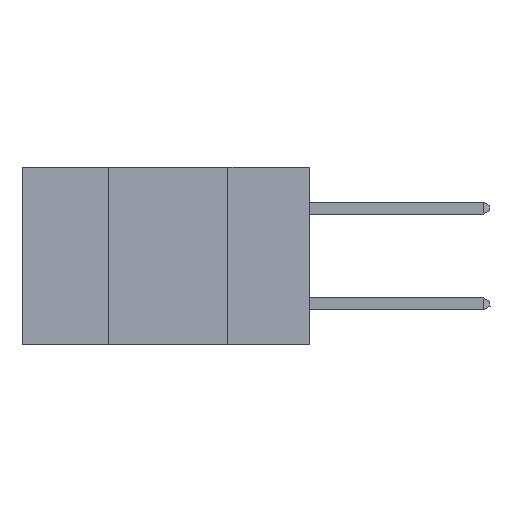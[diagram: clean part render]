
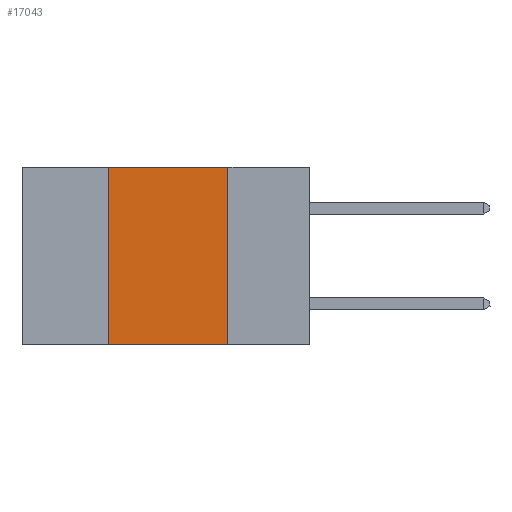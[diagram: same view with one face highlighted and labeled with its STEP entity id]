
A CAD part, left-side view. The second image highlights one B-rep face of the part: STEP entity #17043.
In plain terms, the highlighted planar face has unit normal (-1, 0, 0).
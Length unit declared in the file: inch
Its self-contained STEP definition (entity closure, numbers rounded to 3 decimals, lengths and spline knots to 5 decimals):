
#282 = FACE_OUTER_BOUND ( 'NONE', #10484, .T. ) ;
#453 = ORIENTED_EDGE ( 'NONE', *, *, #3353, .F. ) ;
#843 = EDGE_CURVE ( 'NONE', #7472, #19707, #16392, .T. ) ;
#1840 = VERTEX_POINT ( 'NONE', #17248 ) ;
#2102 = CARTESIAN_POINT ( 'NONE',  ( 0., 0.17, -0.37 ) ) ;
#2778 = CARTESIAN_POINT ( 'NONE',  ( 0., 0.6, -0.37 ) ) ;
#2872 = DIRECTION ( 'NONE',  ( 0., -1., 0. ) ) ;
#3353 = EDGE_CURVE ( 'NONE', #7472, #11350, #10577, .T. ) ;
#3792 = LINE ( 'NONE', #11026, #17487 ) ;
#5064 = CARTESIAN_POINT ( 'NONE',  ( 0., 0.42, 0. ) ) ;
#6886 = DIRECTION ( 'NONE',  ( 0., 0., 1. ) ) ;
#7207 = EDGE_CURVE ( 'NONE', #1840, #19707, #3792, .T. ) ;
#7472 = VERTEX_POINT ( 'NONE', #20380 ) ;
#7990 = DIRECTION ( 'NONE',  ( 1., 0., 0. ) ) ;
#9653 = ORIENTED_EDGE ( 'NONE', *, *, #18401, .F. ) ;
#10167 = CARTESIAN_POINT ( 'NONE',  ( 0., 0.6, 0. ) ) ;
#10215 = ORIENTED_EDGE ( 'NONE', *, *, #843, .T. ) ;
#10484 = EDGE_LOOP ( 'NONE', ( #23046, #9653, #453, #10215 ) ) ;
#10577 = LINE ( 'NONE', #5064, #19283 ) ;
#11026 = CARTESIAN_POINT ( 'NONE',  ( 0., 0.17, 0. ) ) ;
#11350 = VERTEX_POINT ( 'NONE', #15951 ) ;
#11531 = CARTESIAN_POINT ( 'NONE',  ( 0., 0.6, 0. ) ) ;
#12777 = DIRECTION ( 'NONE',  ( 0., 0., -1. ) ) ;
#15951 = CARTESIAN_POINT ( 'NONE',  ( 0., 0.42, 0. ) ) ;
#16392 = LINE ( 'NONE', #2778, #20456 ) ;
#16795 = PLANE ( 'NONE',  #18494 ) ;
#17043 = ADVANCED_FACE ( 'NONE', ( #282 ), #16795, .F. ) ;
#17248 = CARTESIAN_POINT ( 'NONE',  ( 0., 0.17, 0. ) ) ;
#17487 = VECTOR ( 'NONE', #12777, 39.37008 ) ;
#18401 = EDGE_CURVE ( 'NONE', #11350, #1840, #22032, .T. ) ;
#18494 = AXIS2_PLACEMENT_3D ( 'NONE', #11531, #7990, #20276 ) ;
#19283 = VECTOR ( 'NONE', #6886, 39.37008 ) ;
#19549 = VECTOR ( 'NONE', #2872, 39.37008 ) ;
#19707 = VERTEX_POINT ( 'NONE', #2102 ) ;
#20276 = DIRECTION ( 'NONE',  ( 0., 0., -1. ) ) ;
#20380 = CARTESIAN_POINT ( 'NONE',  ( 0., 0.42, -0.37 ) ) ;
#20456 = VECTOR ( 'NONE', #21717, 39.37008 ) ;
#21717 = DIRECTION ( 'NONE',  ( 0., -1., 0. ) ) ;
#22032 = LINE ( 'NONE', #10167, #19549 ) ;
#23046 = ORIENTED_EDGE ( 'NONE', *, *, #7207, .F. ) ;
